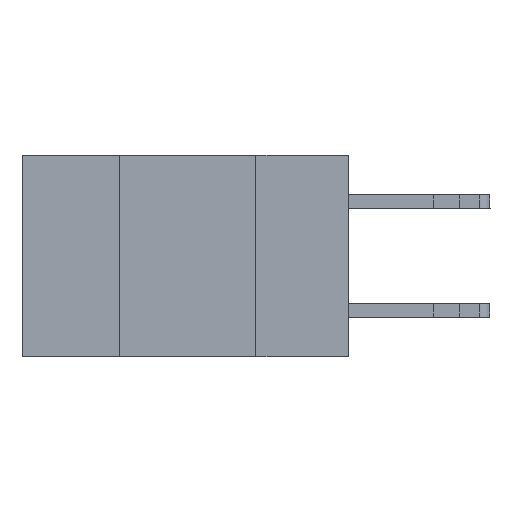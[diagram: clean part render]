
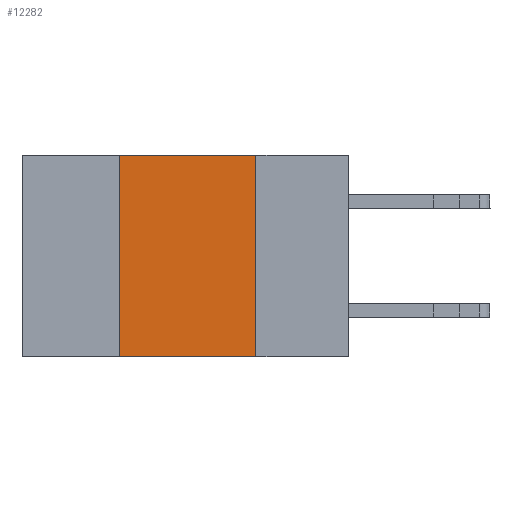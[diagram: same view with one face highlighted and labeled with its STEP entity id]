
A CAD part, left-side view. The second image highlights one B-rep face of the part: STEP entity #12282.
In plain terms, the highlighted planar face has unit normal (-1, 0, 0).
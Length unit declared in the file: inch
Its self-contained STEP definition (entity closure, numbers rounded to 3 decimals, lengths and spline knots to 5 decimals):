
#2451 = ORIENTED_EDGE ( 'NONE', *, *, #9147, .F. ) ;
#3170 = VERTEX_POINT ( 'NONE', #3528 ) ;
#3207 = VECTOR ( 'NONE', #6600, 39.37008 ) ;
#3512 = EDGE_LOOP ( 'NONE', ( #2451, #6169, #6176, #4734 ) ) ;
#3514 = DIRECTION ( 'NONE',  ( 0., 0., 1. ) ) ;
#3528 = CARTESIAN_POINT ( 'NONE',  ( 0., 0.42, -0.37 ) ) ;
#3749 = VECTOR ( 'NONE', #3807, 39.37008 ) ;
#3807 = DIRECTION ( 'NONE',  ( 0., -1., 0. ) ) ;
#3824 = VERTEX_POINT ( 'NONE', #7297 ) ;
#4504 = CARTESIAN_POINT ( 'NONE',  ( 0., 0.6, 0. ) ) ;
#4734 = ORIENTED_EDGE ( 'NONE', *, *, #14026, .T. ) ;
#4826 = CARTESIAN_POINT ( 'NONE',  ( 0., 0.6, 0. ) ) ;
#5865 = LINE ( 'NONE', #12157, #11589 ) ;
#6087 = LINE ( 'NONE', #4826, #3749 ) ;
#6134 = EDGE_CURVE ( 'NONE', #3170, #3824, #5865, .T. ) ;
#6169 = ORIENTED_EDGE ( 'NONE', *, *, #11319, .F. ) ;
#6176 = ORIENTED_EDGE ( 'NONE', *, *, #6134, .F. ) ;
#6207 = CARTESIAN_POINT ( 'NONE',  ( 0., 0.17, 0. ) ) ;
#6248 = VERTEX_POINT ( 'NONE', #9601 ) ;
#6600 = DIRECTION ( 'NONE',  ( 0., -1., 0. ) ) ;
#6973 = AXIS2_PLACEMENT_3D ( 'NONE', #4504, #13299, #9502 ) ;
#6979 = FACE_OUTER_BOUND ( 'NONE', #3512, .T. ) ;
#6980 = VECTOR ( 'NONE', #8830, 39.37008 ) ;
#7297 = CARTESIAN_POINT ( 'NONE',  ( 0., 0.42, 0. ) ) ;
#8510 = LINE ( 'NONE', #12524, #6980 ) ;
#8830 = DIRECTION ( 'NONE',  ( 0., 0., -1. ) ) ;
#9147 = EDGE_CURVE ( 'NONE', #11644, #6248, #8510, .T. ) ;
#9502 = DIRECTION ( 'NONE',  ( 0., 0., -1. ) ) ;
#9601 = CARTESIAN_POINT ( 'NONE',  ( 0., 0.17, -0.37 ) ) ;
#11319 = EDGE_CURVE ( 'NONE', #3824, #11644, #6087, .T. ) ;
#11589 = VECTOR ( 'NONE', #3514, 39.37008 ) ;
#11644 = VERTEX_POINT ( 'NONE', #6207 ) ;
#12157 = CARTESIAN_POINT ( 'NONE',  ( 0., 0.42, -0.37 ) ) ;
#12282 = ADVANCED_FACE ( 'NONE', ( #6979 ), #15780, .F. ) ;
#12524 = CARTESIAN_POINT ( 'NONE',  ( 0., 0.17, -0.37 ) ) ;
#13299 = DIRECTION ( 'NONE',  ( 1., 0., 0. ) ) ;
#13927 = CARTESIAN_POINT ( 'NONE',  ( 0., 0.6, -0.37 ) ) ;
#14026 = EDGE_CURVE ( 'NONE', #3170, #6248, #15403, .T. ) ;
#15403 = LINE ( 'NONE', #13927, #3207 ) ;
#15780 = PLANE ( 'NONE',  #6973 ) ;
